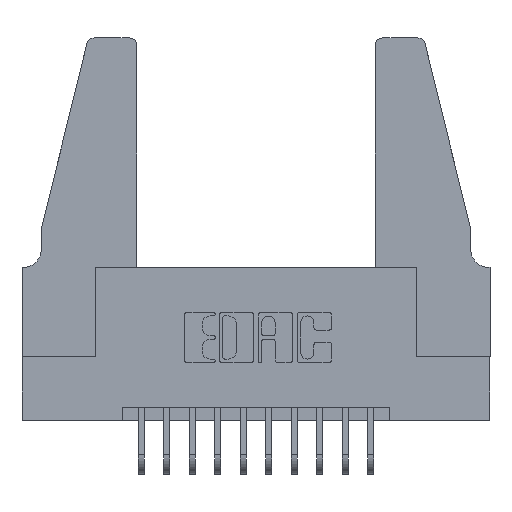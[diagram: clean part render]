
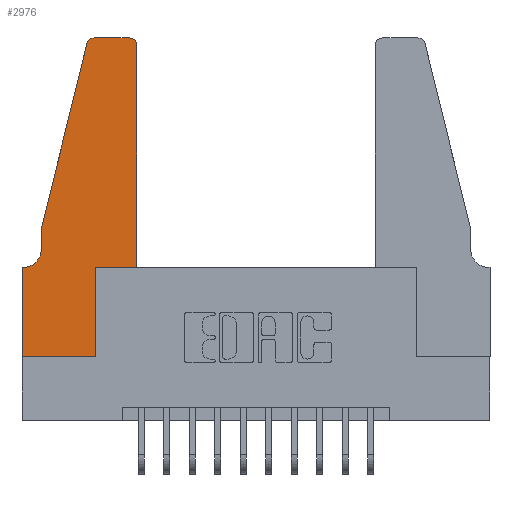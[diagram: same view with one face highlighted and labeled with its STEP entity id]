
A CAD part, top view. The second image highlights one B-rep face of the part: STEP entity #2976.
In plain terms, the highlighted planar face has unit normal (0, 0, 1).
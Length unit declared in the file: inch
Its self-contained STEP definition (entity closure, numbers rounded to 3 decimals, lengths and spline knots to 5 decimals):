
#125 = DIRECTION ( 'NONE',  ( 0., 1., 0. ) ) ;
#146 = DIRECTION ( 'NONE',  ( 0., 0., 1. ) ) ;
#270 = ORIENTED_EDGE ( 'NONE', *, *, #4238, .T. ) ;
#476 = DIRECTION ( 'NONE',  ( -1., 0., 0. ) ) ;
#532 = CARTESIAN_POINT ( 'NONE',  ( 0.0755, 0.5, 0.37 ) ) ;
#621 = ORIENTED_EDGE ( 'NONE', *, *, #786, .T. ) ;
#622 = CARTESIAN_POINT ( 'NONE',  ( 0.0755, 0.5, 0.37 ) ) ;
#753 = CARTESIAN_POINT ( 'NONE',  ( 0.0055, 0.35, 0.37 ) ) ;
#769 = VERTEX_POINT ( 'NONE', #2825 ) ;
#786 = EDGE_CURVE ( 'NONE', #10903, #1276, #13654, .T. ) ;
#818 = ORIENTED_EDGE ( 'NONE', *, *, #3547, .T. ) ;
#870 = VERTEX_POINT ( 'NONE', #3667 ) ;
#879 = DIRECTION ( 'NONE',  ( 1., 0., 0. ) ) ;
#1171 = CARTESIAN_POINT ( 'NONE',  ( 0., 0.35, 0.37 ) ) ;
#1176 = VECTOR ( 'NONE', #12549, 39.37008 ) ;
#1276 = VERTEX_POINT ( 'NONE', #1171 ) ;
#1404 = CARTESIAN_POINT ( 'NONE',  ( 0.0755, 0.42, 0.37 ) ) ;
#1500 = ORIENTED_EDGE ( 'NONE', *, *, #11024, .T. ) ;
#1509 = ORIENTED_EDGE ( 'NONE', *, *, #12506, .T. ) ;
#1584 = LINE ( 'NONE', #6568, #1176 ) ;
#1693 = LINE ( 'NONE', #532, #11340 ) ;
#1900 = EDGE_CURVE ( 'NONE', #870, #11484, #15609, .T. ) ;
#2237 = VECTOR ( 'NONE', #4320, 39.37008 ) ;
#2358 = CARTESIAN_POINT ( 'NONE',  ( 0.4505, 0.35, 0.37 ) ) ;
#2825 = CARTESIAN_POINT ( 'NONE',  ( 0.284, 1.25, 0.37 ) ) ;
#2976 = ADVANCED_FACE ( 'NONE', ( #10431 ), #5990, .T. ) ;
#3085 = VERTEX_POINT ( 'NONE', #2358 ) ;
#3176 = DIRECTION ( 'NONE',  ( 0., 0., -1. ) ) ;
#3310 = EDGE_CURVE ( 'NONE', #769, #870, #14980, .T. ) ;
#3440 = DIRECTION ( 'NONE',  ( 0., 0., 1. ) ) ;
#3547 = EDGE_CURVE ( 'NONE', #11484, #14564, #1693, .T. ) ;
#3667 = CARTESIAN_POINT ( 'NONE',  ( 0.25487, 1.22718, 0.37 ) ) ;
#3871 = CARTESIAN_POINT ( 'NONE',  ( 0.0755, 0.35, 0.37 ) ) ;
#3934 = LINE ( 'NONE', #9639, #11541 ) ;
#4029 = EDGE_CURVE ( 'NONE', #3085, #9902, #5613, .T. ) ;
#4128 = CARTESIAN_POINT ( 'NONE',  ( 0.4205, 1.25, 0.37 ) ) ;
#4238 = EDGE_CURVE ( 'NONE', #14564, #10903, #9830, .T. ) ;
#4320 = DIRECTION ( 'NONE',  ( -0.239, -0.971, 0. ) ) ;
#4376 = VECTOR ( 'NONE', #476, 39.37008 ) ;
#4475 = ORIENTED_EDGE ( 'NONE', *, *, #4029, .T. ) ;
#4631 = VERTEX_POINT ( 'NONE', #4128 ) ;
#5380 = ORIENTED_EDGE ( 'NONE', *, *, #1900, .T. ) ;
#5578 = EDGE_CURVE ( 'NONE', #12564, #11386, #3934, .T. ) ;
#5613 = LINE ( 'NONE', #9105, #8897 ) ;
#5737 = LINE ( 'NONE', #12257, #14906 ) ;
#5990 = PLANE ( 'NONE',  #12927 ) ;
#6156 = VECTOR ( 'NONE', #10547, 39.37008 ) ;
#6269 = CIRCLE ( 'NONE', #14692, 0.03 ) ;
#6568 = CARTESIAN_POINT ( 'NONE',  ( 0.2865, 0.35, 0.37 ) ) ;
#7099 = DIRECTION ( 'NONE',  ( 0., -1., 0. ) ) ;
#7461 = DIRECTION ( 'NONE',  ( 1., 0., 0. ) ) ;
#7478 = CARTESIAN_POINT ( 'NONE',  ( 0., 0., 0.37 ) ) ;
#7575 = CARTESIAN_POINT ( 'NONE',  ( 0.0755, 0.5, 0.37 ) ) ;
#7588 = ORIENTED_EDGE ( 'NONE', *, *, #7607, .T. ) ;
#7607 = EDGE_CURVE ( 'NONE', #11386, #13693, #1584, .T. ) ;
#7779 = ORIENTED_EDGE ( 'NONE', *, *, #5578, .T. ) ;
#7914 = CARTESIAN_POINT ( 'NONE',  ( 0.284, 1.22, 0.37 ) ) ;
#8494 = DIRECTION ( 'NONE',  ( 1., 0., 0. ) ) ;
#8508 = CARTESIAN_POINT ( 'NONE',  ( 0., 0.35, 0.37 ) ) ;
#8529 = VECTOR ( 'NONE', #7461, 39.37008 ) ;
#8603 = DIRECTION ( 'NONE',  ( 0., 0., 1. ) ) ;
#8646 = ORIENTED_EDGE ( 'NONE', *, *, #10172, .T. ) ;
#8694 = AXIS2_PLACEMENT_3D ( 'NONE', #10680, #3176, #11848 ) ;
#8897 = VECTOR ( 'NONE', #125, 39.37008 ) ;
#8904 = LINE ( 'NONE', #9839, #8529 ) ;
#9105 = CARTESIAN_POINT ( 'NONE',  ( 0.4505, 0.35, 0.37 ) ) ;
#9123 = DIRECTION ( 'NONE',  ( 1., 0., 0. ) ) ;
#9178 = EDGE_CURVE ( 'NONE', #13693, #3085, #8904, .T. ) ;
#9331 = CARTESIAN_POINT ( 'NONE',  ( 0.2605, 1.25, 0.37 ) ) ;
#9639 = CARTESIAN_POINT ( 'NONE',  ( 0., 0., 0.37 ) ) ;
#9830 = CIRCLE ( 'NONE', #8694, 0.07 ) ;
#9839 = CARTESIAN_POINT ( 'NONE',  ( 0.4505, 0.35, 0.37 ) ) ;
#9902 = VERTEX_POINT ( 'NONE', #11182 ) ;
#10172 = EDGE_CURVE ( 'NONE', #4631, #769, #15658, .T. ) ;
#10179 = ORIENTED_EDGE ( 'NONE', *, *, #3310, .T. ) ;
#10277 = EDGE_LOOP ( 'NONE', ( #8646, #10179, #5380, #818, #270, #621, #1500, #7779, #7588, #15571, #4475, #1509 ) ) ;
#10431 = FACE_OUTER_BOUND ( 'NONE', #10277, .T. ) ;
#10547 = DIRECTION ( 'NONE',  ( -1., 0., 0. ) ) ;
#10680 = CARTESIAN_POINT ( 'NONE',  ( 0.0055, 0.42, 0.37 ) ) ;
#10903 = VERTEX_POINT ( 'NONE', #753 ) ;
#11024 = EDGE_CURVE ( 'NONE', #1276, #12564, #5737, .T. ) ;
#11091 = AXIS2_PLACEMENT_3D ( 'NONE', #7914, #146, #9123 ) ;
#11157 = DIRECTION ( 'NONE',  ( 0., -1., 0. ) ) ;
#11182 = CARTESIAN_POINT ( 'NONE',  ( 0.4505, 1.22, 0.37 ) ) ;
#11340 = VECTOR ( 'NONE', #7099, 39.37008 ) ;
#11386 = VERTEX_POINT ( 'NONE', #14077 ) ;
#11484 = VERTEX_POINT ( 'NONE', #622 ) ;
#11541 = VECTOR ( 'NONE', #8494, 39.37008 ) ;
#11848 = DIRECTION ( 'NONE',  ( -1., 0., 0. ) ) ;
#12075 = DIRECTION ( 'NONE',  ( 1., 0., 0. ) ) ;
#12257 = CARTESIAN_POINT ( 'NONE',  ( 0., 0., 0.37 ) ) ;
#12506 = EDGE_CURVE ( 'NONE', #9902, #4631, #6269, .T. ) ;
#12549 = DIRECTION ( 'NONE',  ( 0., 1., 0. ) ) ;
#12564 = VERTEX_POINT ( 'NONE', #7478 ) ;
#12927 = AXIS2_PLACEMENT_3D ( 'NONE', #8508, #3440, #12075 ) ;
#13654 = LINE ( 'NONE', #3871, #4376 ) ;
#13693 = VERTEX_POINT ( 'NONE', #15444 ) ;
#14077 = CARTESIAN_POINT ( 'NONE',  ( 0.2865, 0., 0.37 ) ) ;
#14564 = VERTEX_POINT ( 'NONE', #1404 ) ;
#14692 = AXIS2_PLACEMENT_3D ( 'NONE', #15631, #8603, #879 ) ;
#14906 = VECTOR ( 'NONE', #11157, 39.37008 ) ;
#14980 = CIRCLE ( 'NONE', #11091, 0.03 ) ;
#15444 = CARTESIAN_POINT ( 'NONE',  ( 0.2865, 0.35, 0.37 ) ) ;
#15571 = ORIENTED_EDGE ( 'NONE', *, *, #9178, .T. ) ;
#15609 = LINE ( 'NONE', #7575, #2237 ) ;
#15631 = CARTESIAN_POINT ( 'NONE',  ( 0.4205, 1.22, 0.37 ) ) ;
#15658 = LINE ( 'NONE', #9331, #6156 ) ;
